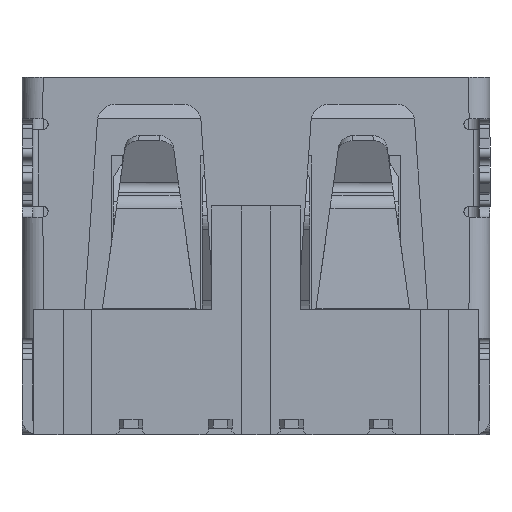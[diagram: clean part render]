
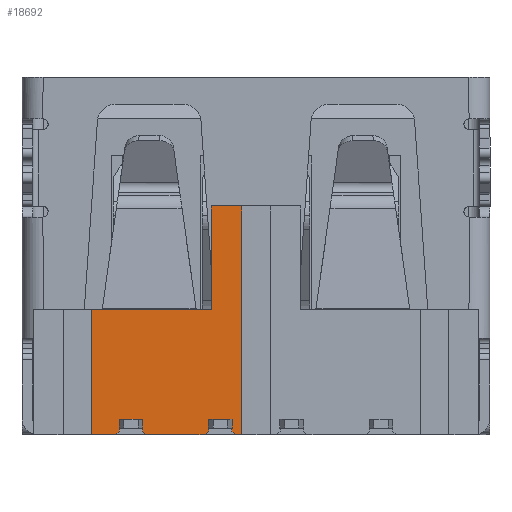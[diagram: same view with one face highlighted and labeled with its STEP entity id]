
A CAD part, front view. The second image highlights one B-rep face of the part: STEP entity #18692.
In plain terms, the highlighted face is planar.
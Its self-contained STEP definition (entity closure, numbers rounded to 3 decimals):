
#30 = CARTESIAN_POINT ( 'NONE',  ( -88.943, -6.807, 5. ) ) ;
#42 = CARTESIAN_POINT ( 'NONE',  ( -87.118, -6.807, 0.15 ) ) ;
#471 = CARTESIAN_POINT ( 'NONE',  ( -88.993, -6.807, 4.95 ) ) ;
#554 = ORIENTED_EDGE ( 'NONE', *, *, #17366, .T. ) ;
#714 = VECTOR ( 'NONE', #10302, 1000. ) ;
#987 = CARTESIAN_POINT ( 'NONE',  ( -86.868, -6.807, 4.57 ) ) ;
#1174 = DIRECTION ( 'NONE',  ( 1., 0., 0. ) ) ;
#1210 = VERTEX_POINT ( 'NONE', #9616 ) ;
#1505 = EDGE_CURVE ( 'NONE', #1210, #9965, #22805, .T. ) ;
#1547 = VERTEX_POINT ( 'NONE', #10732 ) ;
#1588 = DIRECTION ( 'NONE',  ( 1., 0., 0. ) ) ;
#1624 = ORIENTED_EDGE ( 'NONE', *, *, #17748, .T. ) ;
#1666 = CARTESIAN_POINT ( 'NONE',  ( -89.043, -6.807, 4.9 ) ) ;
#1695 = CARTESIAN_POINT ( 'NONE',  ( -86.543, -6.807, 4.57 ) ) ;
#1761 = EDGE_CURVE ( 'NONE', #1885, #22826, #18828, .T. ) ;
#1823 = LINE ( 'NONE', #17120, #7680 ) ;
#1885 = VERTEX_POINT ( 'NONE', #2429 ) ;
#1909 = ORIENTED_EDGE ( 'NONE', *, *, #8215, .T. ) ;
#1949 = VECTOR ( 'NONE', #2524, 1000. ) ;
#2082 = DIRECTION ( 'NONE',  ( 0., 0., 1. ) ) ;
#2374 = CARTESIAN_POINT ( 'NONE',  ( -87.193, -6.807, 4.57 ) ) ;
#2429 = CARTESIAN_POINT ( 'NONE',  ( -89.693, -6.807, 4.9 ) ) ;
#2524 = DIRECTION ( 'NONE',  ( 0.707, 0., -0.707 ) ) ;
#2594 = LINE ( 'NONE', #6643, #714 ) ;
#3092 = EDGE_CURVE ( 'NONE', #4822, #6688, #12235, .T. ) ;
#3146 = FACE_OUTER_BOUND ( 'NONE', #8586, .T. ) ;
#3277 = VERTEX_POINT ( 'NONE', #1695 ) ;
#3532 = ORIENTED_EDGE ( 'NONE', *, *, #10493, .T. ) ;
#3567 = LINE ( 'NONE', #18255, #8646 ) ;
#3807 = ORIENTED_EDGE ( 'NONE', *, *, #7404, .T. ) ;
#4102 = CARTESIAN_POINT ( 'NONE',  ( -86.268, -6.807, 1.8 ) ) ;
#4346 = VERTEX_POINT ( 'NONE', #21368 ) ;
#4382 = CARTESIAN_POINT ( 'NONE',  ( -87.118, -6.807, -1.4 ) ) ;
#4386 = CARTESIAN_POINT ( 'NONE',  ( -90.468, -6.807, 1.5 ) ) ;
#4407 = DIRECTION ( 'NONE',  ( 0., 0., 1. ) ) ;
#4543 = CARTESIAN_POINT ( 'NONE',  ( -89.605, -6.807, 1.5 ) ) ;
#4652 = VERTEX_POINT ( 'NONE', #30 ) ;
#4775 = CARTESIAN_POINT ( 'NONE',  ( -86.868, -6.807, -1.4 ) ) ;
#4822 = VERTEX_POINT ( 'NONE', #13634 ) ;
#6122 = LINE ( 'NONE', #21168, #19928 ) ;
#6132 = VERTEX_POINT ( 'NONE', #14117 ) ;
#6377 = EDGE_CURVE ( 'NONE', #19964, #4652, #17615, .T. ) ;
#6579 = DIRECTION ( 'NONE',  ( 0., 1., 0. ) ) ;
#6630 = ORIENTED_EDGE ( 'NONE', *, *, #20059, .T. ) ;
#6643 = CARTESIAN_POINT ( 'NONE',  ( -85.868, -6.807, 5. ) ) ;
#6688 = VERTEX_POINT ( 'NONE', #4386 ) ;
#6854 = EDGE_CURVE ( 'NONE', #9965, #15447, #12878, .T. ) ;
#7075 = PLANE ( 'NONE',  #7359 ) ;
#7077 = EDGE_CURVE ( 'NONE', #3277, #6132, #15697, .T. ) ;
#7181 = CARTESIAN_POINT ( 'NONE',  ( -90.468, -6.807, 5. ) ) ;
#7294 = ORIENTED_EDGE ( 'NONE', *, *, #10976, .T. ) ;
#7359 = AXIS2_PLACEMENT_3D ( 'NONE', #10725, #6579, #18190 ) ;
#7404 = EDGE_CURVE ( 'NONE', #7669, #4346, #1823, .T. ) ;
#7669 = VERTEX_POINT ( 'NONE', #7181 ) ;
#7680 = VECTOR ( 'NONE', #18720, 1000. ) ;
#7699 = ORIENTED_EDGE ( 'NONE', *, *, #11387, .T. ) ;
#8021 = DIRECTION ( 'NONE',  ( 0., 0., -1. ) ) ;
#8071 = LINE ( 'NONE', #19210, #19486 ) ;
#8215 = EDGE_CURVE ( 'NONE', #1547, #11363, #12109, .T. ) ;
#8319 = DIRECTION ( 'NONE',  ( 0.707, 0., 0.707 ) ) ;
#8389 = ORIENTED_EDGE ( 'NONE', *, *, #1505, .T. ) ;
#8586 = EDGE_LOOP ( 'NONE', ( #6630, #1909, #19267, #13944, #7294, #3807, #7699, #22028, #554, #3532, #18951, #1624, #8389, #21640, #21728, #23851, #21641, #16350 ) ) ;
#8646 = VECTOR ( 'NONE', #11030, 1000. ) ;
#9616 = CARTESIAN_POINT ( 'NONE',  ( -87.293, -6.807, 5. ) ) ;
#9965 = VERTEX_POINT ( 'NONE', #23837 ) ;
#10130 = VECTOR ( 'NONE', #8021, 1000. ) ;
#10302 = DIRECTION ( 'NONE',  ( 1., 0., 0. ) ) ;
#10387 = CARTESIAN_POINT ( 'NONE',  ( -89.693, -6.807, 4.57 ) ) ;
#10474 = VECTOR ( 'NONE', #23149, 1000. ) ;
#10493 = EDGE_CURVE ( 'NONE', #18917, #19964, #18854, .T. ) ;
#10725 = CARTESIAN_POINT ( 'NONE',  ( -87.492, -6.807, -1.528 ) ) ;
#10732 = CARTESIAN_POINT ( 'NONE',  ( -86.268, -6.807, -1.4 ) ) ;
#10892 = CARTESIAN_POINT ( 'NONE',  ( -89.368, -6.807, 4.57 ) ) ;
#10976 = EDGE_CURVE ( 'NONE', #6688, #7669, #6122, .T. ) ;
#11030 = DIRECTION ( 'NONE',  ( 0.707, 0., 0.707 ) ) ;
#11203 = VERTEX_POINT ( 'NONE', #14767 ) ;
#11326 = CARTESIAN_POINT ( 'NONE',  ( -89.043, -6.807, 4.57 ) ) ;
#11363 = VERTEX_POINT ( 'NONE', #4382 ) ;
#11387 = EDGE_CURVE ( 'NONE', #4346, #1885, #17221, .T. ) ;
#12109 = LINE ( 'NONE', #4775, #10474 ) ;
#12235 = LINE ( 'NONE', #4543, #13178 ) ;
#12878 = LINE ( 'NONE', #20096, #18975 ) ;
#12949 = EDGE_CURVE ( 'NONE', #11363, #4822, #16831, .T. ) ;
#13067 = VERTEX_POINT ( 'NONE', #19024 ) ;
#13080 = VECTOR ( 'NONE', #23276, 1000. ) ;
#13178 = VECTOR ( 'NONE', #17379, 1000. ) ;
#13347 = CARTESIAN_POINT ( 'NONE',  ( -89.043, -6.807, 4.613 ) ) ;
#13563 = EDGE_CURVE ( 'NONE', #15447, #3277, #19830, .T. ) ;
#13634 = CARTESIAN_POINT ( 'NONE',  ( -87.118, -6.807, 1.5 ) ) ;
#13944 = ORIENTED_EDGE ( 'NONE', *, *, #3092, .T. ) ;
#14117 = CARTESIAN_POINT ( 'NONE',  ( -86.543, -6.807, 4.9 ) ) ;
#14708 = DIRECTION ( 'NONE',  ( 0., 0., -1. ) ) ;
#14767 = CARTESIAN_POINT ( 'NONE',  ( -86.443, -6.807, 5. ) ) ;
#14984 = DIRECTION ( 'NONE',  ( 0., 0., 1. ) ) ;
#15447 = VERTEX_POINT ( 'NONE', #2374 ) ;
#15632 = VECTOR ( 'NONE', #8319, 1000. ) ;
#15697 = LINE ( 'NONE', #19346, #13080 ) ;
#16161 = VECTOR ( 'NONE', #21089, 1000. ) ;
#16350 = ORIENTED_EDGE ( 'NONE', *, *, #19540, .T. ) ;
#16538 = VECTOR ( 'NONE', #22139, 1000. ) ;
#16831 = LINE ( 'NONE', #42, #19773 ) ;
#17111 = VECTOR ( 'NONE', #1588, 1000. ) ;
#17120 = CARTESIAN_POINT ( 'NONE',  ( -90.943, -6.807, 5. ) ) ;
#17221 = LINE ( 'NONE', #23110, #1949 ) ;
#17366 = EDGE_CURVE ( 'NONE', #22826, #18917, #20183, .T. ) ;
#17379 = DIRECTION ( 'NONE',  ( -1., 0., 0. ) ) ;
#17615 = LINE ( 'NONE', #471, #15632 ) ;
#17748 = EDGE_CURVE ( 'NONE', #4652, #1210, #8071, .T. ) ;
#17750 = DIRECTION ( 'NONE',  ( 1., 0., 0. ) ) ;
#18190 = DIRECTION ( 'NONE',  ( 0., 0., 1. ) ) ;
#18255 = CARTESIAN_POINT ( 'NONE',  ( -86.493, -6.807, 4.95 ) ) ;
#18692 = ADVANCED_FACE ( 'NONE', ( #3146 ), #7075, .T. ) ;
#18720 = DIRECTION ( 'NONE',  ( 1., 0., 0. ) ) ;
#18828 = LINE ( 'NONE', #22260, #16538 ) ;
#18854 = LINE ( 'NONE', #13347, #19126 ) ;
#18917 = VERTEX_POINT ( 'NONE', #11326 ) ;
#18951 = ORIENTED_EDGE ( 'NONE', *, *, #6377, .T. ) ;
#18975 = VECTOR ( 'NONE', #14708, 1000. ) ;
#19024 = CARTESIAN_POINT ( 'NONE',  ( -86.268, -6.807, 5. ) ) ;
#19126 = VECTOR ( 'NONE', #2082, 1000. ) ;
#19210 = CARTESIAN_POINT ( 'NONE',  ( -88.118, -6.807, 5. ) ) ;
#19267 = ORIENTED_EDGE ( 'NONE', *, *, #12949, .T. ) ;
#19346 = CARTESIAN_POINT ( 'NONE',  ( -86.543, -6.807, 4.613 ) ) ;
#19486 = VECTOR ( 'NONE', #1174, 1000. ) ;
#19540 = EDGE_CURVE ( 'NONE', #11203, #13067, #2594, .T. ) ;
#19773 = VECTOR ( 'NONE', #14984, 1000. ) ;
#19830 = LINE ( 'NONE', #987, #20179 ) ;
#19928 = VECTOR ( 'NONE', #4407, 1000. ) ;
#19964 = VERTEX_POINT ( 'NONE', #1666 ) ;
#20059 = EDGE_CURVE ( 'NONE', #13067, #1547, #21240, .T. ) ;
#20096 = CARTESIAN_POINT ( 'NONE',  ( -87.193, -6.807, 4.613 ) ) ;
#20179 = VECTOR ( 'NONE', #17750, 1000. ) ;
#20183 = LINE ( 'NONE', #10892, #17111 ) ;
#20718 = CARTESIAN_POINT ( 'NONE',  ( -87.243, -6.807, 4.95 ) ) ;
#21089 = DIRECTION ( 'NONE',  ( 0.707, 0., -0.707 ) ) ;
#21168 = CARTESIAN_POINT ( 'NONE',  ( -90.468, -6.807, 3.25 ) ) ;
#21240 = LINE ( 'NONE', #4102, #10130 ) ;
#21368 = CARTESIAN_POINT ( 'NONE',  ( -89.793, -6.807, 5. ) ) ;
#21640 = ORIENTED_EDGE ( 'NONE', *, *, #6854, .T. ) ;
#21641 = ORIENTED_EDGE ( 'NONE', *, *, #21885, .T. ) ;
#21728 = ORIENTED_EDGE ( 'NONE', *, *, #13563, .T. ) ;
#21885 = EDGE_CURVE ( 'NONE', #6132, #11203, #3567, .T. ) ;
#22028 = ORIENTED_EDGE ( 'NONE', *, *, #1761, .T. ) ;
#22139 = DIRECTION ( 'NONE',  ( 0., 0., -1. ) ) ;
#22260 = CARTESIAN_POINT ( 'NONE',  ( -89.693, -6.807, 4.735 ) ) ;
#22805 = LINE ( 'NONE', #20718, #16161 ) ;
#22826 = VERTEX_POINT ( 'NONE', #10387 ) ;
#23110 = CARTESIAN_POINT ( 'NONE',  ( -89.743, -6.807, 4.95 ) ) ;
#23149 = DIRECTION ( 'NONE',  ( -1., 0., 0. ) ) ;
#23276 = DIRECTION ( 'NONE',  ( 0., 0., 1. ) ) ;
#23837 = CARTESIAN_POINT ( 'NONE',  ( -87.193, -6.807, 4.9 ) ) ;
#23851 = ORIENTED_EDGE ( 'NONE', *, *, #7077, .T. ) ;
